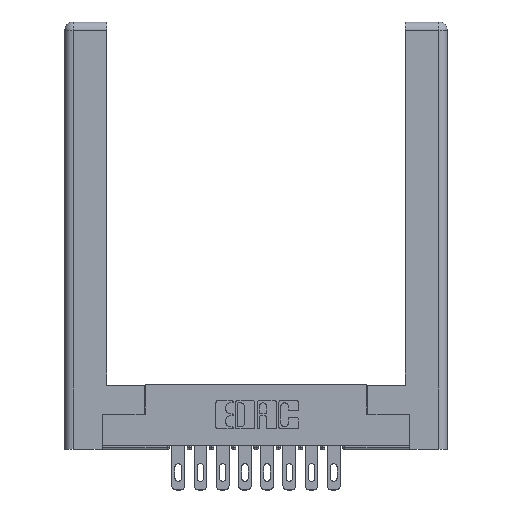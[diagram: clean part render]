
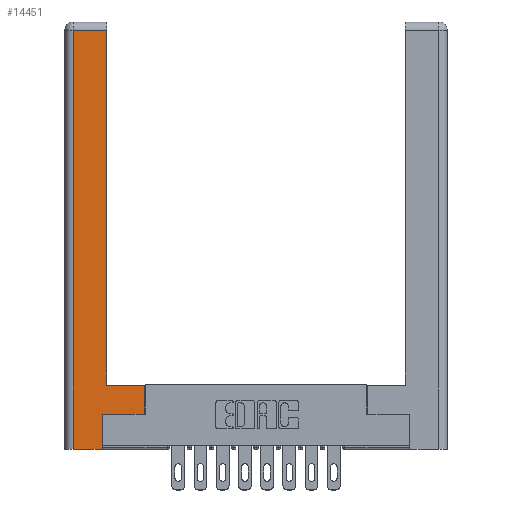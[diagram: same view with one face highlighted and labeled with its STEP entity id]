
A CAD part, top view. The second image highlights one B-rep face of the part: STEP entity #14451.
In plain terms, the highlighted planar face has unit normal (0, 0, 1).
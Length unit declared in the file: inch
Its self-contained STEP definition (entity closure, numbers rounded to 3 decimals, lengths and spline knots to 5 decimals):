
#219 = LINE ( 'NONE', #14782, #12551 ) ;
#822 = PLANE ( 'NONE',  #14912 ) ;
#1174 = CARTESIAN_POINT ( 'NONE',  ( 0.295, 0.45, 0. ) ) ;
#1300 = ORIENTED_EDGE ( 'NONE', *, *, #15453, .T. ) ;
#1455 = VERTEX_POINT ( 'NONE', #10130 ) ;
#1492 = VECTOR ( 'NONE', #3116, 39.37008 ) ;
#1693 = VECTOR ( 'NONE', #4034, 39.37008 ) ;
#1906 = LINE ( 'NONE', #11208, #9176 ) ;
#2002 = EDGE_CURVE ( 'NONE', #8612, #5771, #4589, .T. ) ;
#2031 = VERTEX_POINT ( 'NONE', #11837 ) ;
#2238 = CARTESIAN_POINT ( 'NONE',  ( 0.565, 0.245, 0. ) ) ;
#2757 = CARTESIAN_POINT ( 'NONE',  ( 0.295, 2.94, 0. ) ) ;
#3075 = ORIENTED_EDGE ( 'NONE', *, *, #15354, .T. ) ;
#3116 = DIRECTION ( 'NONE',  ( -1., 0., 0. ) ) ;
#3317 = CARTESIAN_POINT ( 'NONE',  ( 0., 0., 0. ) ) ;
#3339 = ORIENTED_EDGE ( 'NONE', *, *, #11850, .T. ) ;
#4034 = DIRECTION ( 'NONE',  ( 0., 1., 0. ) ) ;
#4104 = ORIENTED_EDGE ( 'NONE', *, *, #9528, .T. ) ;
#4221 = CARTESIAN_POINT ( 'NONE',  ( 0.0615, 2.94, 0. ) ) ;
#4589 = LINE ( 'NONE', #4594, #9019 ) ;
#4594 = CARTESIAN_POINT ( 'NONE',  ( 0.265, 0., 0. ) ) ;
#5133 = DIRECTION ( 'NONE',  ( 0., 1., 0. ) ) ;
#5234 = DIRECTION ( 'NONE',  ( -1., 0., 0. ) ) ;
#5576 = VECTOR ( 'NONE', #5808, 39.37008 ) ;
#5634 = EDGE_CURVE ( 'NONE', #13260, #2031, #14602, .T. ) ;
#5771 = VERTEX_POINT ( 'NONE', #12227 ) ;
#5776 = LINE ( 'NONE', #11640, #5576 ) ;
#5781 = DIRECTION ( 'NONE',  ( 1., 0., 0. ) ) ;
#5808 = DIRECTION ( 'NONE',  ( 1., 0., 0. ) ) ;
#5986 = ORIENTED_EDGE ( 'NONE', *, *, #2002, .T. ) ;
#5995 = LINE ( 'NONE', #7438, #7101 ) ;
#6615 = VERTEX_POINT ( 'NONE', #1174 ) ;
#7101 = VECTOR ( 'NONE', #5133, 39.37008 ) ;
#7438 = CARTESIAN_POINT ( 'NONE',  ( 0.295, 3., 0. ) ) ;
#7781 = ORIENTED_EDGE ( 'NONE', *, *, #10510, .T. ) ;
#7903 = DIRECTION ( 'NONE',  ( 0., 0., -1. ) ) ;
#7946 = DIRECTION ( 'NONE',  ( -1., 0., 0. ) ) ;
#8137 = ORIENTED_EDGE ( 'NONE', *, *, #5634, .T. ) ;
#8612 = VERTEX_POINT ( 'NONE', #10386 ) ;
#8648 = DIRECTION ( 'NONE',  ( 0., -1., 0. ) ) ;
#9019 = VECTOR ( 'NONE', #5781, 39.37008 ) ;
#9176 = VECTOR ( 'NONE', #5234, 39.37008 ) ;
#9528 = EDGE_CURVE ( 'NONE', #11390, #1455, #13860, .T. ) ;
#10045 = EDGE_LOOP ( 'NONE', ( #7781, #8137, #12381, #5986, #1300, #3339, #4104, #3075 ) ) ;
#10130 = CARTESIAN_POINT ( 'NONE',  ( 0.565, 0.45, 0. ) ) ;
#10386 = CARTESIAN_POINT ( 'NONE',  ( 0.0615, 0., 0. ) ) ;
#10510 = EDGE_CURVE ( 'NONE', #6615, #13260, #5995, .T. ) ;
#10885 = FACE_OUTER_BOUND ( 'NONE', #10045, .T. ) ;
#11003 = EDGE_CURVE ( 'NONE', #2031, #8612, #14586, .T. ) ;
#11009 = CARTESIAN_POINT ( 'NONE',  ( 0.0615, 0., 0. ) ) ;
#11208 = CARTESIAN_POINT ( 'NONE',  ( 0.295, 0.45, 0. ) ) ;
#11390 = VERTEX_POINT ( 'NONE', #2238 ) ;
#11395 = VECTOR ( 'NONE', #8648, 39.37008 ) ;
#11584 = VERTEX_POINT ( 'NONE', #11739 ) ;
#11640 = CARTESIAN_POINT ( 'NONE',  ( 0.565, 0.245, 0. ) ) ;
#11739 = CARTESIAN_POINT ( 'NONE',  ( 0.265, 0.245, 0. ) ) ;
#11837 = CARTESIAN_POINT ( 'NONE',  ( 0.0615, 2.94, 0. ) ) ;
#11850 = EDGE_CURVE ( 'NONE', #11584, #11390, #5776, .T. ) ;
#12227 = CARTESIAN_POINT ( 'NONE',  ( 0.265, 0., 0. ) ) ;
#12381 = ORIENTED_EDGE ( 'NONE', *, *, #11003, .T. ) ;
#12551 = VECTOR ( 'NONE', #13485, 39.37008 ) ;
#13260 = VERTEX_POINT ( 'NONE', #2757 ) ;
#13485 = DIRECTION ( 'NONE',  ( 0., 1., 0. ) ) ;
#13860 = LINE ( 'NONE', #14808, #1693 ) ;
#14451 = ADVANCED_FACE ( 'NONE', ( #10885 ), #822, .F. ) ;
#14586 = LINE ( 'NONE', #11009, #11395 ) ;
#14602 = LINE ( 'NONE', #4221, #1492 ) ;
#14782 = CARTESIAN_POINT ( 'NONE',  ( 0.265, 0.245, 0. ) ) ;
#14808 = CARTESIAN_POINT ( 'NONE',  ( 0.565, 0.45, 0. ) ) ;
#14912 = AXIS2_PLACEMENT_3D ( 'NONE', #3317, #7903, #7946 ) ;
#15354 = EDGE_CURVE ( 'NONE', #1455, #6615, #1906, .T. ) ;
#15453 = EDGE_CURVE ( 'NONE', #5771, #11584, #219, .T. ) ;
